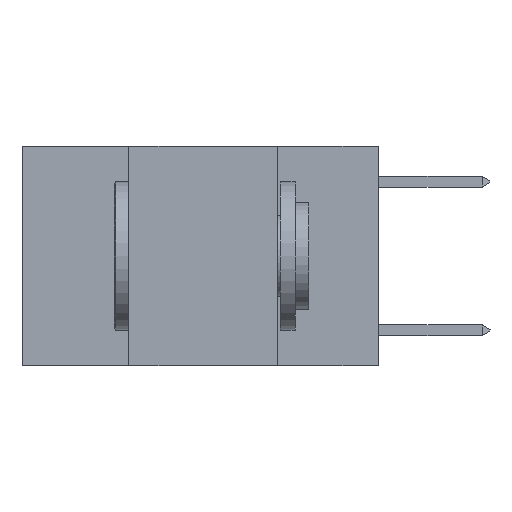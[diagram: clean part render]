
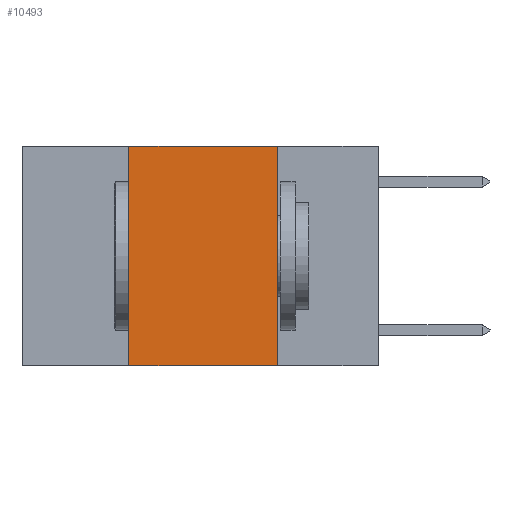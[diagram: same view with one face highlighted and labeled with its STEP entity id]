
A CAD part, left-side view. The second image highlights one B-rep face of the part: STEP entity #10493.
In plain terms, the highlighted planar face has unit normal (-1, 0, 0).
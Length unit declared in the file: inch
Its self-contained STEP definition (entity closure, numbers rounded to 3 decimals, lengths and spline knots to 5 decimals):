
#365 = VECTOR ( 'NONE', #11250, 39.37008 ) ;
#823 = ORIENTED_EDGE ( 'NONE', *, *, #7872, .T. ) ;
#3340 = LINE ( 'NONE', #16502, #10439 ) ;
#3356 = CARTESIAN_POINT ( 'NONE',  ( 0., 0.6, 0. ) ) ;
#4184 = CARTESIAN_POINT ( 'NONE',  ( 0., 0.17, 0. ) ) ;
#4701 = VERTEX_POINT ( 'NONE', #12424 ) ;
#4798 = EDGE_CURVE ( 'NONE', #14934, #7470, #12196, .T. ) ;
#6219 = PLANE ( 'NONE',  #7111 ) ;
#6931 = DIRECTION ( 'NONE',  ( 0., -1., 0. ) ) ;
#7068 = CARTESIAN_POINT ( 'NONE',  ( 0., 0.42, -0.37 ) ) ;
#7111 = AXIS2_PLACEMENT_3D ( 'NONE', #3356, #7666, #17135 ) ;
#7277 = LINE ( 'NONE', #16984, #10576 ) ;
#7427 = CARTESIAN_POINT ( 'NONE',  ( 0., 0.42, 0. ) ) ;
#7470 = VERTEX_POINT ( 'NONE', #14971 ) ;
#7666 = DIRECTION ( 'NONE',  ( 1., 0., 0. ) ) ;
#7872 = EDGE_CURVE ( 'NONE', #13175, #7470, #7277, .T. ) ;
#8850 = DIRECTION ( 'NONE',  ( 0., 0., 1. ) ) ;
#9103 = CARTESIAN_POINT ( 'NONE',  ( 0., 0.17, 0. ) ) ;
#9718 = EDGE_CURVE ( 'NONE', #4701, #14934, #3340, .T. ) ;
#10439 = VECTOR ( 'NONE', #6931, 39.37008 ) ;
#10493 = ADVANCED_FACE ( 'NONE', ( #16509 ), #6219, .F. ) ;
#10576 = VECTOR ( 'NONE', #11747, 39.37008 ) ;
#11235 = VECTOR ( 'NONE', #8850, 39.37008 ) ;
#11250 = DIRECTION ( 'NONE',  ( 0., 0., -1. ) ) ;
#11369 = ORIENTED_EDGE ( 'NONE', *, *, #4798, .F. ) ;
#11686 = LINE ( 'NONE', #7427, #11235 ) ;
#11747 = DIRECTION ( 'NONE',  ( 0., -1., 0. ) ) ;
#11871 = EDGE_CURVE ( 'NONE', #13175, #4701, #11686, .T. ) ;
#12196 = LINE ( 'NONE', #4184, #365 ) ;
#12424 = CARTESIAN_POINT ( 'NONE',  ( 0., 0.42, 0. ) ) ;
#12475 = ORIENTED_EDGE ( 'NONE', *, *, #11871, .F. ) ;
#13175 = VERTEX_POINT ( 'NONE', #7068 ) ;
#14934 = VERTEX_POINT ( 'NONE', #9103 ) ;
#14971 = CARTESIAN_POINT ( 'NONE',  ( 0., 0.17, -0.37 ) ) ;
#16502 = CARTESIAN_POINT ( 'NONE',  ( 0., 0.6, 0. ) ) ;
#16509 = FACE_OUTER_BOUND ( 'NONE', #17716, .T. ) ;
#16984 = CARTESIAN_POINT ( 'NONE',  ( 0., 0.6, -0.37 ) ) ;
#17135 = DIRECTION ( 'NONE',  ( 0., 0., -1. ) ) ;
#17535 = ORIENTED_EDGE ( 'NONE', *, *, #9718, .F. ) ;
#17716 = EDGE_LOOP ( 'NONE', ( #11369, #17535, #12475, #823 ) ) ;
